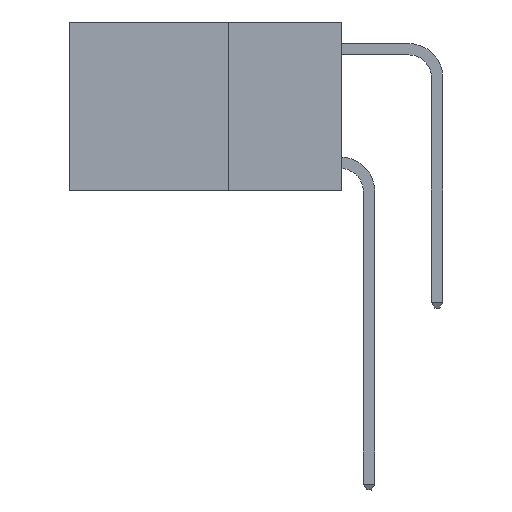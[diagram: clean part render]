
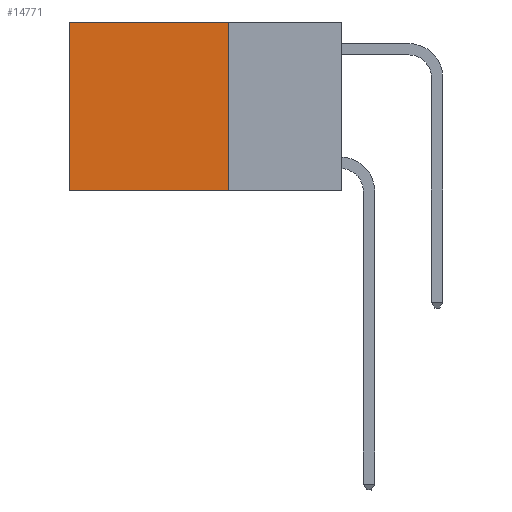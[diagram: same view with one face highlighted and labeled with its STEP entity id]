
A CAD part, left-side view. The second image highlights one B-rep face of the part: STEP entity #14771.
In plain terms, the highlighted planar face has unit normal (-1, 0, 0).
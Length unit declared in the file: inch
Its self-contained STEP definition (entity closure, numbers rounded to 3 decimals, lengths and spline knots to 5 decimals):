
#1743 = CARTESIAN_POINT ( 'NONE',  ( 0.2625, 0.25, 0. ) ) ;
#1773 = LINE ( 'NONE', #9611, #30725 ) ;
#3204 = LINE ( 'NONE', #26118, #19501 ) ;
#5291 = VECTOR ( 'NONE', #16799, 39.37008 ) ;
#5620 = VERTEX_POINT ( 'NONE', #27922 ) ;
#6474 = EDGE_CURVE ( 'NONE', #5620, #20752, #1773, .T. ) ;
#9181 = CARTESIAN_POINT ( 'NONE',  ( 0.2625, 0.25, -0.37 ) ) ;
#9489 = AXIS2_PLACEMENT_3D ( 'NONE', #23961, #19309, #12096 ) ;
#9611 = CARTESIAN_POINT ( 'NONE',  ( 0.2625, 0.25, 0. ) ) ;
#11623 = PLANE ( 'NONE',  #9489 ) ;
#12096 = DIRECTION ( 'NONE',  ( 0., 0., -1. ) ) ;
#12713 = ORIENTED_EDGE ( 'NONE', *, *, #6474, .T. ) ;
#12911 = VECTOR ( 'NONE', #25655, 39.37008 ) ;
#13566 = DIRECTION ( 'NONE',  ( 0., 0., -1. ) ) ;
#13627 = LINE ( 'NONE', #1743, #5291 ) ;
#14771 = ADVANCED_FACE ( 'NONE', ( #30091 ), #11623, .F. ) ;
#15628 = CARTESIAN_POINT ( 'NONE',  ( 0.2625, 0.25, -0.37 ) ) ;
#16799 = DIRECTION ( 'NONE',  ( 0., 0., -1. ) ) ;
#17065 = CARTESIAN_POINT ( 'NONE',  ( 0.2625, 0.6, -0.37 ) ) ;
#17533 = EDGE_CURVE ( 'NONE', #5620, #32741, #13627, .T. ) ;
#18608 = VERTEX_POINT ( 'NONE', #17065 ) ;
#18781 = CARTESIAN_POINT ( 'NONE',  ( 0.2625, 0.6, 0. ) ) ;
#19309 = DIRECTION ( 'NONE',  ( 1., 0., 0. ) ) ;
#19501 = VECTOR ( 'NONE', #13566, 39.37008 ) ;
#20286 = ORIENTED_EDGE ( 'NONE', *, *, #22003, .F. ) ;
#20752 = VERTEX_POINT ( 'NONE', #18781 ) ;
#21428 = DIRECTION ( 'NONE',  ( 0., 1., 0. ) ) ;
#22003 = EDGE_CURVE ( 'NONE', #32741, #18608, #32778, .T. ) ;
#22441 = ORIENTED_EDGE ( 'NONE', *, *, #17533, .F. ) ;
#23961 = CARTESIAN_POINT ( 'NONE',  ( 0.2625, 0.25, 0. ) ) ;
#25086 = EDGE_CURVE ( 'NONE', #20752, #18608, #3204, .T. ) ;
#25655 = DIRECTION ( 'NONE',  ( 0., 1., 0. ) ) ;
#26118 = CARTESIAN_POINT ( 'NONE',  ( 0.2625, 0.6, 0. ) ) ;
#26320 = EDGE_LOOP ( 'NONE', ( #29250, #20286, #22441, #12713 ) ) ;
#27922 = CARTESIAN_POINT ( 'NONE',  ( 0.2625, 0.25, 0. ) ) ;
#29250 = ORIENTED_EDGE ( 'NONE', *, *, #25086, .T. ) ;
#30091 = FACE_OUTER_BOUND ( 'NONE', #26320, .T. ) ;
#30725 = VECTOR ( 'NONE', #21428, 39.37008 ) ;
#32741 = VERTEX_POINT ( 'NONE', #9181 ) ;
#32778 = LINE ( 'NONE', #15628, #12911 ) ;
